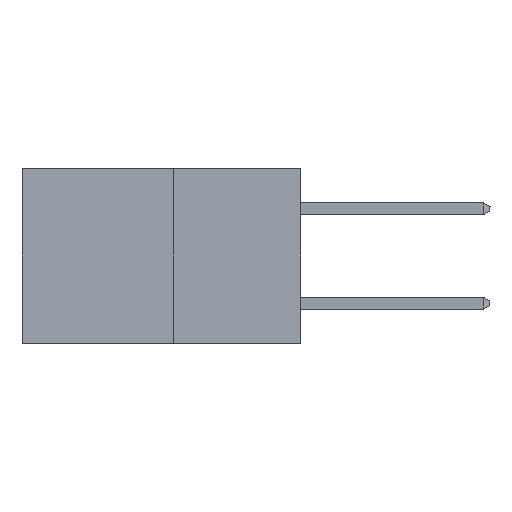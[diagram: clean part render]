
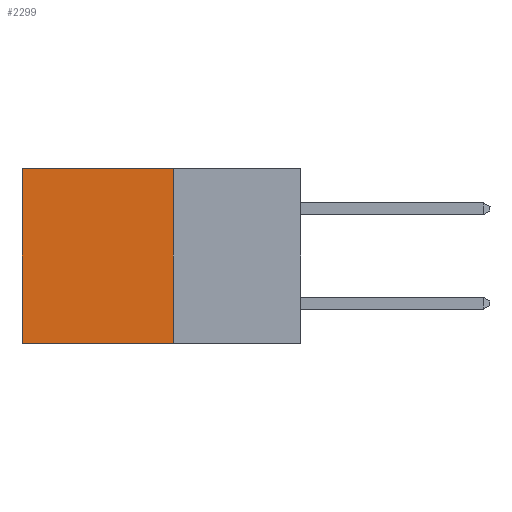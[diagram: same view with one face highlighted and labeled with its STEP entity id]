
A CAD part, left-side view. The second image highlights one B-rep face of the part: STEP entity #2299.
In plain terms, the highlighted planar face has unit normal (-1, 0, 0).
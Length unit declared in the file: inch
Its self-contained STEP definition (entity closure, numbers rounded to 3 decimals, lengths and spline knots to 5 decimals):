
#651 = CARTESIAN_POINT ( 'NONE',  ( 0.277, 0.27, -0.37 ) ) ;
#800 = VECTOR ( 'NONE', #3949, 39.37008 ) ;
#1067 = ORIENTED_EDGE ( 'NONE', *, *, #1721, .T. ) ;
#1721 = EDGE_CURVE ( 'NONE', #6270, #2045, #7153, .T. ) ;
#1964 = EDGE_CURVE ( 'NONE', #7080, #2435, #7243, .T. ) ;
#2045 = VERTEX_POINT ( 'NONE', #8893 ) ;
#2243 = DIRECTION ( 'NONE',  ( 0., 0., -1. ) ) ;
#2299 = ADVANCED_FACE ( 'NONE', ( #7660 ), #2609, .F. ) ;
#2389 = CARTESIAN_POINT ( 'NONE',  ( 0.277, 0.27, -0.37 ) ) ;
#2435 = VERTEX_POINT ( 'NONE', #7473 ) ;
#2440 = ORIENTED_EDGE ( 'NONE', *, *, #2902, .T. ) ;
#2465 = CARTESIAN_POINT ( 'NONE',  ( 0.277, 0.27, -0.37 ) ) ;
#2609 = PLANE ( 'NONE',  #6180 ) ;
#2902 = EDGE_CURVE ( 'NONE', #2045, #2435, #8139, .T. ) ;
#2970 = ORIENTED_EDGE ( 'NONE', *, *, #1964, .F. ) ;
#3224 = CARTESIAN_POINT ( 'NONE',  ( 0.277, 0.27, 0. ) ) ;
#3247 = ORIENTED_EDGE ( 'NONE', *, *, #4454, .F. ) ;
#3702 = VECTOR ( 'NONE', #8327, 39.37008 ) ;
#3853 = DIRECTION ( 'NONE',  ( 1., 0., 0. ) ) ;
#3880 = DIRECTION ( 'NONE',  ( 0., 0., -1. ) ) ;
#3949 = DIRECTION ( 'NONE',  ( 0., 0., -1. ) ) ;
#4079 = CARTESIAN_POINT ( 'NONE',  ( 0.277, 0.27, -0.37 ) ) ;
#4442 = DIRECTION ( 'NONE',  ( 0., 1., 0. ) ) ;
#4454 = EDGE_CURVE ( 'NONE', #6270, #7080, #5242, .T. ) ;
#5242 = LINE ( 'NONE', #2389, #6752 ) ;
#5944 = CARTESIAN_POINT ( 'NONE',  ( 0.277, 0.59, -0.37 ) ) ;
#6180 = AXIS2_PLACEMENT_3D ( 'NONE', #4079, #3853, #3880 ) ;
#6270 = VERTEX_POINT ( 'NONE', #6888 ) ;
#6752 = VECTOR ( 'NONE', #2243, 39.37008 ) ;
#6876 = VECTOR ( 'NONE', #4442, 39.37008 ) ;
#6888 = CARTESIAN_POINT ( 'NONE',  ( 0.277, 0.27, 0. ) ) ;
#7080 = VERTEX_POINT ( 'NONE', #651 ) ;
#7153 = LINE ( 'NONE', #3224, #3702 ) ;
#7243 = LINE ( 'NONE', #2465, #6876 ) ;
#7473 = CARTESIAN_POINT ( 'NONE',  ( 0.277, 0.59, -0.37 ) ) ;
#7660 = FACE_OUTER_BOUND ( 'NONE', #8489, .T. ) ;
#8139 = LINE ( 'NONE', #5944, #800 ) ;
#8327 = DIRECTION ( 'NONE',  ( 0., 1., 0. ) ) ;
#8489 = EDGE_LOOP ( 'NONE', ( #2440, #2970, #3247, #1067 ) ) ;
#8893 = CARTESIAN_POINT ( 'NONE',  ( 0.277, 0.59, 0. ) ) ;
